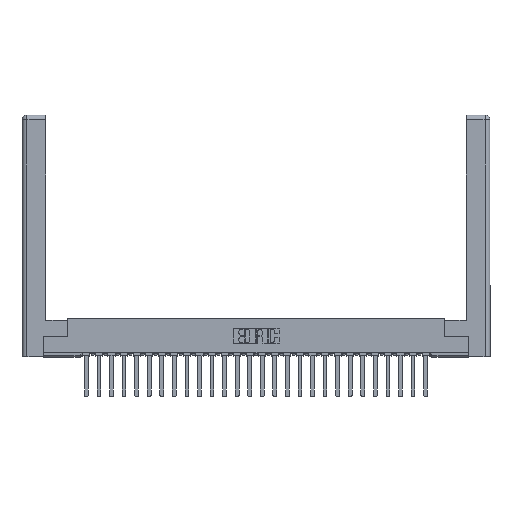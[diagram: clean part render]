
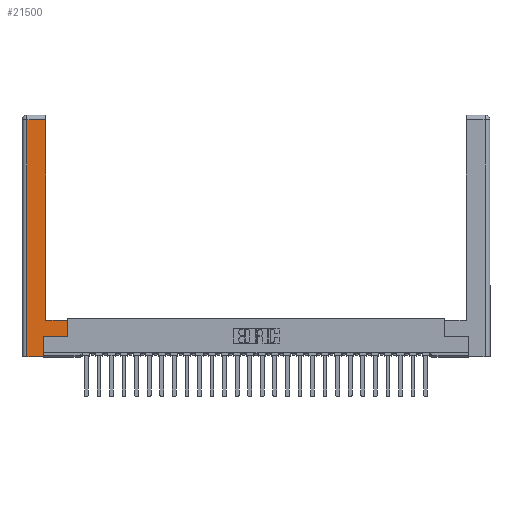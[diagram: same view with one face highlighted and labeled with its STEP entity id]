
A CAD part, top view. The second image highlights one B-rep face of the part: STEP entity #21500.
In plain terms, the highlighted planar face has unit normal (0, 0, 1).
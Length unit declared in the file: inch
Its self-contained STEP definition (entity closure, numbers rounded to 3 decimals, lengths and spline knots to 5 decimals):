
#434 = CARTESIAN_POINT ( 'NONE',  ( 0.295, 2.94, 0. ) ) ;
#1079 = ORIENTED_EDGE ( 'NONE', *, *, #12492, .T. ) ;
#1198 = CARTESIAN_POINT ( 'NONE',  ( 0.265, 0., 0. ) ) ;
#1782 = VECTOR ( 'NONE', #17821, 39.37008 ) ;
#1891 = LINE ( 'NONE', #8795, #11377 ) ;
#2508 = VECTOR ( 'NONE', #4320, 39.37008 ) ;
#2822 = VECTOR ( 'NONE', #15766, 39.37008 ) ;
#2994 = VERTEX_POINT ( 'NONE', #22972 ) ;
#3648 = EDGE_CURVE ( 'NONE', #18156, #2994, #1891, .T. ) ;
#3706 = LINE ( 'NONE', #1198, #13275 ) ;
#4006 = CARTESIAN_POINT ( 'NONE',  ( 0.265, 0., 0. ) ) ;
#4261 = ORIENTED_EDGE ( 'NONE', *, *, #18605, .T. ) ;
#4320 = DIRECTION ( 'NONE',  ( 0., 1., 0. ) ) ;
#4742 = CARTESIAN_POINT ( 'NONE',  ( 0.565, 0.45, 0. ) ) ;
#4980 = LINE ( 'NONE', #14244, #12840 ) ;
#5362 = AXIS2_PLACEMENT_3D ( 'NONE', #11637, #27407, #7240 ) ;
#5545 = EDGE_CURVE ( 'NONE', #8369, #9447, #26982, .T. ) ;
#5616 = EDGE_CURVE ( 'NONE', #2994, #8724, #22401, .T. ) ;
#5835 = EDGE_CURVE ( 'NONE', #19550, #28854, #3706, .T. ) ;
#5836 = DIRECTION ( 'NONE',  ( 0., 1., 0. ) ) ;
#5950 = DIRECTION ( 'NONE',  ( 0., -1., 0. ) ) ;
#6101 = LINE ( 'NONE', #25670, #23938 ) ;
#6284 = LINE ( 'NONE', #28509, #12089 ) ;
#6802 = CARTESIAN_POINT ( 'NONE',  ( 0.295, 3., 0. ) ) ;
#7240 = DIRECTION ( 'NONE',  ( -1., 0., 0. ) ) ;
#7420 = CARTESIAN_POINT ( 'NONE',  ( 0.0615, 0., 0. ) ) ;
#8369 = VERTEX_POINT ( 'NONE', #18752 ) ;
#8644 = DIRECTION ( 'NONE',  ( 1., 0., 0. ) ) ;
#8699 = CARTESIAN_POINT ( 'NONE',  ( 0.295, 0.45, 0. ) ) ;
#8724 = VERTEX_POINT ( 'NONE', #11789 ) ;
#8795 = CARTESIAN_POINT ( 'NONE',  ( 0.565, 0.245, 0. ) ) ;
#9316 = FACE_OUTER_BOUND ( 'NONE', #11889, .T. ) ;
#9447 = VERTEX_POINT ( 'NONE', #434 ) ;
#11377 = VECTOR ( 'NONE', #8644, 39.37008 ) ;
#11532 = ORIENTED_EDGE ( 'NONE', *, *, #5835, .T. ) ;
#11637 = CARTESIAN_POINT ( 'NONE',  ( 0., 0., 0. ) ) ;
#11789 = CARTESIAN_POINT ( 'NONE',  ( 0.565, 0.45, 0. ) ) ;
#11889 = EDGE_LOOP ( 'NONE', ( #13476, #4261, #25219, #11532, #1079, #12868, #16123, #23238 ) ) ;
#12089 = VECTOR ( 'NONE', #5836, 39.37008 ) ;
#12492 = EDGE_CURVE ( 'NONE', #28854, #18156, #6284, .T. ) ;
#12506 = DIRECTION ( 'NONE',  ( 1., 0., 0. ) ) ;
#12840 = VECTOR ( 'NONE', #22801, 39.37008 ) ;
#12868 = ORIENTED_EDGE ( 'NONE', *, *, #3648, .T. ) ;
#13275 = VECTOR ( 'NONE', #12506, 39.37008 ) ;
#13432 = PLANE ( 'NONE',  #5362 ) ;
#13476 = ORIENTED_EDGE ( 'NONE', *, *, #5545, .T. ) ;
#14244 = CARTESIAN_POINT ( 'NONE',  ( 0.0615, 2.94, 0. ) ) ;
#15181 = EDGE_CURVE ( 'NONE', #19737, #19550, #6101, .T. ) ;
#15766 = DIRECTION ( 'NONE',  ( 0., 1., 0. ) ) ;
#16123 = ORIENTED_EDGE ( 'NONE', *, *, #5616, .T. ) ;
#17546 = CARTESIAN_POINT ( 'NONE',  ( 0.0615, 2.94, 0. ) ) ;
#17821 = DIRECTION ( 'NONE',  ( -1., 0., 0. ) ) ;
#18156 = VERTEX_POINT ( 'NONE', #24642 ) ;
#18605 = EDGE_CURVE ( 'NONE', #9447, #19737, #4980, .T. ) ;
#18752 = CARTESIAN_POINT ( 'NONE',  ( 0.295, 0.45, 0. ) ) ;
#19550 = VERTEX_POINT ( 'NONE', #7420 ) ;
#19737 = VERTEX_POINT ( 'NONE', #17546 ) ;
#21500 = ADVANCED_FACE ( 'NONE', ( #9316 ), #13432, .F. ) ;
#22230 = LINE ( 'NONE', #8699, #1782 ) ;
#22401 = LINE ( 'NONE', #4742, #2508 ) ;
#22801 = DIRECTION ( 'NONE',  ( -1., 0., 0. ) ) ;
#22972 = CARTESIAN_POINT ( 'NONE',  ( 0.565, 0.245, 0. ) ) ;
#23238 = ORIENTED_EDGE ( 'NONE', *, *, #25936, .T. ) ;
#23938 = VECTOR ( 'NONE', #5950, 39.37008 ) ;
#24642 = CARTESIAN_POINT ( 'NONE',  ( 0.265, 0.245, 0. ) ) ;
#25219 = ORIENTED_EDGE ( 'NONE', *, *, #15181, .T. ) ;
#25670 = CARTESIAN_POINT ( 'NONE',  ( 0.0615, 0., 0. ) ) ;
#25936 = EDGE_CURVE ( 'NONE', #8724, #8369, #22230, .T. ) ;
#26982 = LINE ( 'NONE', #6802, #2822 ) ;
#27407 = DIRECTION ( 'NONE',  ( 0., 0., -1. ) ) ;
#28509 = CARTESIAN_POINT ( 'NONE',  ( 0.265, 0.245, 0. ) ) ;
#28854 = VERTEX_POINT ( 'NONE', #4006 ) ;
